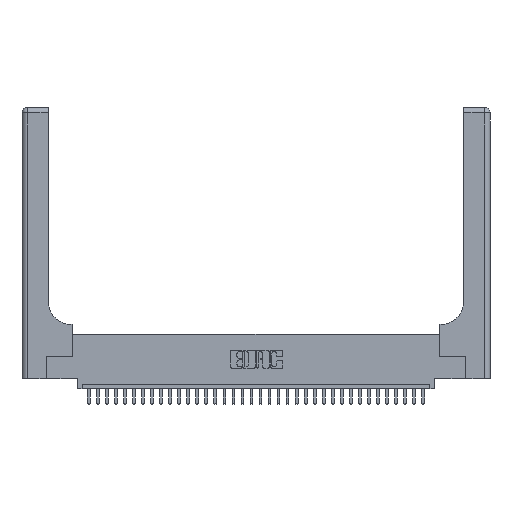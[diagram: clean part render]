
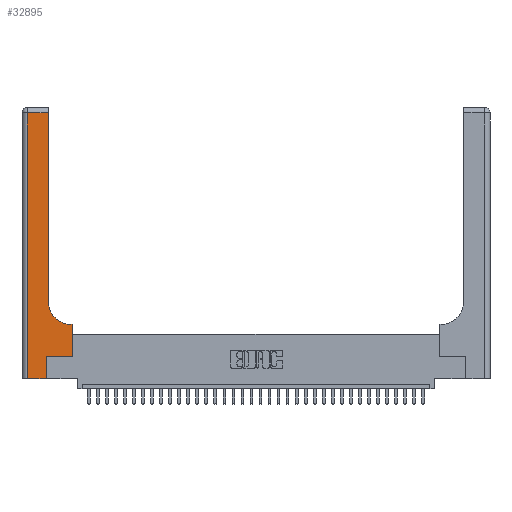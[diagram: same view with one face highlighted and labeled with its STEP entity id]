
A CAD part, top view. The second image highlights one B-rep face of the part: STEP entity #32895.
In plain terms, the highlighted planar face has unit normal (0, 0, 1).
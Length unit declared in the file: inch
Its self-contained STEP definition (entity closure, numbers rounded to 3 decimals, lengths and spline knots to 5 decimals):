
#88 = AXIS2_PLACEMENT_3D ( 'NONE', #10054, #31679, #5035 ) ;
#657 = EDGE_CURVE ( 'NONE', #23913, #34353, #10372, .T. ) ;
#1018 = EDGE_CURVE ( 'NONE', #14076, #12101, #23726, .T. ) ;
#1698 = ORIENTED_EDGE ( 'NONE', *, *, #32361, .T. ) ;
#1885 = ORIENTED_EDGE ( 'NONE', *, *, #657, .T. ) ;
#1922 = VERTEX_POINT ( 'NONE', #14269 ) ;
#3239 = VECTOR ( 'NONE', #18809, 39.37008 ) ;
#3486 = ORIENTED_EDGE ( 'NONE', *, *, #21984, .T. ) ;
#3617 = CARTESIAN_POINT ( 'NONE',  ( 0.06, 3., 0.37 ) ) ;
#4026 = CARTESIAN_POINT ( 'NONE',  ( 0.2915, 2.94, 0.37 ) ) ;
#4239 = CARTESIAN_POINT ( 'NONE',  ( 0.2915, 0.85, 0.37 ) ) ;
#5035 = DIRECTION ( 'NONE',  ( -1., 0., 0. ) ) ;
#5076 = VECTOR ( 'NONE', #21155, 39.37008 ) ;
#6299 = CARTESIAN_POINT ( 'NONE',  ( 0.06, 0., 0.37 ) ) ;
#6681 = ORIENTED_EDGE ( 'NONE', *, *, #24059, .T. ) ;
#7421 = DIRECTION ( 'NONE',  ( -1., 0., 0. ) ) ;
#8538 = CARTESIAN_POINT ( 'NONE',  ( 0.5415, 0.85, 0.37 ) ) ;
#9170 = FACE_OUTER_BOUND ( 'NONE', #21969, .T. ) ;
#10054 = CARTESIAN_POINT ( 'NONE',  ( 0., 3., 0.37 ) ) ;
#10120 = LINE ( 'NONE', #20729, #15975 ) ;
#10372 = CIRCLE ( 'NONE', #34241, 0.25 ) ;
#11393 = CARTESIAN_POINT ( 'NONE',  ( 0.5415, 0.6, 0.37 ) ) ;
#11399 = ORIENTED_EDGE ( 'NONE', *, *, #18142, .T. ) ;
#11965 = DIRECTION ( 'NONE',  ( 0., 1., 0. ) ) ;
#12101 = VERTEX_POINT ( 'NONE', #28918 ) ;
#12308 = VECTOR ( 'NONE', #24598, 39.37008 ) ;
#13078 = VECTOR ( 'NONE', #30447, 39.37008 ) ;
#13388 = CARTESIAN_POINT ( 'NONE',  ( 0., 0., 0.37 ) ) ;
#13577 = ORIENTED_EDGE ( 'NONE', *, *, #32102, .T. ) ;
#14076 = VERTEX_POINT ( 'NONE', #25060 ) ;
#14115 = DIRECTION ( 'NONE',  ( 1., 0., 0. ) ) ;
#14269 = CARTESIAN_POINT ( 'NONE',  ( 0.5585, 0.6, 0.37 ) ) ;
#14304 = ORIENTED_EDGE ( 'NONE', *, *, #1018, .T. ) ;
#15316 = VERTEX_POINT ( 'NONE', #4026 ) ;
#15975 = VECTOR ( 'NONE', #7421, 39.37008 ) ;
#16117 = CARTESIAN_POINT ( 'NONE',  ( 0.5585, 0.25, 0.37 ) ) ;
#16225 = VECTOR ( 'NONE', #17806, 39.37008 ) ;
#16385 = VERTEX_POINT ( 'NONE', #21311 ) ;
#16632 = VECTOR ( 'NONE', #11965, 39.37008 ) ;
#17806 = DIRECTION ( 'NONE',  ( -1., 0., 0. ) ) ;
#18142 = EDGE_CURVE ( 'NONE', #31815, #1922, #34127, .T. ) ;
#18809 = DIRECTION ( 'NONE',  ( 0., 1., 0. ) ) ;
#19404 = EDGE_CURVE ( 'NONE', #12101, #31815, #19411, .T. ) ;
#19411 = LINE ( 'NONE', #24015, #12308 ) ;
#20312 = LINE ( 'NONE', #29670, #3239 ) ;
#20536 = PLANE ( 'NONE',  #88 ) ;
#20729 = CARTESIAN_POINT ( 'NONE',  ( 0.2915, 0.6, 0.37 ) ) ;
#21155 = DIRECTION ( 'NONE',  ( 1., 0., 0. ) ) ;
#21311 = CARTESIAN_POINT ( 'NONE',  ( 0.06, 2.94, 0.37 ) ) ;
#21969 = EDGE_LOOP ( 'NONE', ( #31842, #6681, #13577, #1698, #14304, #25645, #11399, #3486, #1885 ) ) ;
#21984 = EDGE_CURVE ( 'NONE', #1922, #23913, #10120, .T. ) ;
#22060 = LINE ( 'NONE', #29487, #16225 ) ;
#23694 = VERTEX_POINT ( 'NONE', #6299 ) ;
#23726 = LINE ( 'NONE', #33567, #16632 ) ;
#23913 = VERTEX_POINT ( 'NONE', #11393 ) ;
#24015 = CARTESIAN_POINT ( 'NONE',  ( 0.269, 0.25, 0.37 ) ) ;
#24059 = EDGE_CURVE ( 'NONE', #15316, #16385, #22060, .T. ) ;
#24598 = DIRECTION ( 'NONE',  ( 1., 0., 0. ) ) ;
#24952 = EDGE_CURVE ( 'NONE', #34353, #15316, #20312, .T. ) ;
#25060 = CARTESIAN_POINT ( 'NONE',  ( 0.269, 0., 0.37 ) ) ;
#25248 = DIRECTION ( 'NONE',  ( 0., 1., 0. ) ) ;
#25645 = ORIENTED_EDGE ( 'NONE', *, *, #19404, .T. ) ;
#26991 = VECTOR ( 'NONE', #25248, 39.37008 ) ;
#27253 = DIRECTION ( 'NONE',  ( 0., 0., -1. ) ) ;
#28918 = CARTESIAN_POINT ( 'NONE',  ( 0.269, 0.25, 0.37 ) ) ;
#28934 = CARTESIAN_POINT ( 'NONE',  ( 0.5585, 0.25, 0.37 ) ) ;
#29487 = CARTESIAN_POINT ( 'NONE',  ( 0., 2.94, 0.37 ) ) ;
#29670 = CARTESIAN_POINT ( 'NONE',  ( 0.2915, 3., 0.37 ) ) ;
#30447 = DIRECTION ( 'NONE',  ( 0., -1., 0. ) ) ;
#30565 = LINE ( 'NONE', #13388, #5076 ) ;
#31679 = DIRECTION ( 'NONE',  ( 0., 0., -1. ) ) ;
#31815 = VERTEX_POINT ( 'NONE', #16117 ) ;
#31842 = ORIENTED_EDGE ( 'NONE', *, *, #24952, .T. ) ;
#32102 = EDGE_CURVE ( 'NONE', #16385, #23694, #34348, .T. ) ;
#32361 = EDGE_CURVE ( 'NONE', #23694, #14076, #30565, .T. ) ;
#32895 = ADVANCED_FACE ( 'NONE', ( #9170 ), #20536, .F. ) ;
#33567 = CARTESIAN_POINT ( 'NONE',  ( 0.269, 0., 0.37 ) ) ;
#34127 = LINE ( 'NONE', #28934, #26991 ) ;
#34241 = AXIS2_PLACEMENT_3D ( 'NONE', #8538, #27253, #14115 ) ;
#34348 = LINE ( 'NONE', #3617, #13078 ) ;
#34353 = VERTEX_POINT ( 'NONE', #4239 ) ;
